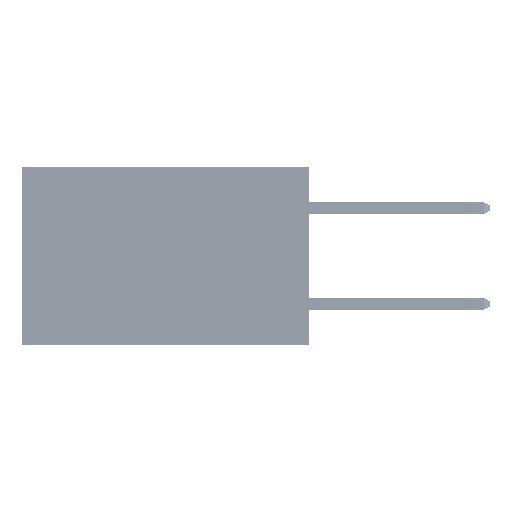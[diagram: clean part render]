
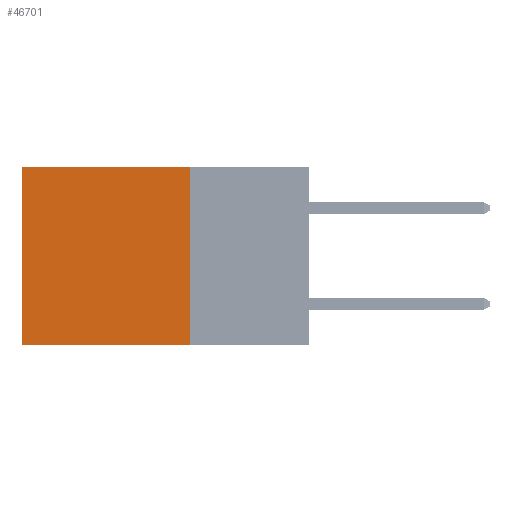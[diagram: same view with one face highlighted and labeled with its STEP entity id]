
A CAD part, left-side view. The second image highlights one B-rep face of the part: STEP entity #46701.
In plain terms, the highlighted planar face has unit normal (-1, 0, 0).
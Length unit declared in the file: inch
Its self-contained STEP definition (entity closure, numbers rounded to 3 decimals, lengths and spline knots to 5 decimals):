
#2729 = DIRECTION ( 'NONE',  ( 0., 0., -1. ) ) ;
#2833 = LINE ( 'NONE', #48284, #40767 ) ;
#3765 = EDGE_CURVE ( 'NONE', #38031, #37282, #28941, .T. ) ;
#4045 = LINE ( 'NONE', #22220, #17287 ) ;
#6251 = DIRECTION ( 'NONE',  ( 0., 0., -1. ) ) ;
#7330 = VERTEX_POINT ( 'NONE', #32236 ) ;
#7373 = VECTOR ( 'NONE', #11178, 39.37008 ) ;
#11178 = DIRECTION ( 'NONE',  ( 0., 1., 0. ) ) ;
#13029 = AXIS2_PLACEMENT_3D ( 'NONE', #47253, #47424, #39059 ) ;
#14104 = EDGE_CURVE ( 'NONE', #38031, #20908, #42827, .T. ) ;
#14466 = ORIENTED_EDGE ( 'NONE', *, *, #3765, .F. ) ;
#15093 = ORIENTED_EDGE ( 'NONE', *, *, #33403, .F. ) ;
#17287 = VECTOR ( 'NONE', #18830, 39.37008 ) ;
#17337 = ORIENTED_EDGE ( 'NONE', *, *, #37130, .T. ) ;
#18830 = DIRECTION ( 'NONE',  ( 0., 1., 0. ) ) ;
#18999 = FACE_OUTER_BOUND ( 'NONE', #23245, .T. ) ;
#19179 = ORIENTED_EDGE ( 'NONE', *, *, #14104, .T. ) ;
#19265 = CARTESIAN_POINT ( 'NONE',  ( 0.2875, 0.6, 0. ) ) ;
#20532 = PLANE ( 'NONE',  #13029 ) ;
#20908 = VERTEX_POINT ( 'NONE', #19265 ) ;
#22220 = CARTESIAN_POINT ( 'NONE',  ( 0.2875, 0.25, -0.37 ) ) ;
#23245 = EDGE_LOOP ( 'NONE', ( #17337, #15093, #14466, #19179 ) ) ;
#25810 = CARTESIAN_POINT ( 'NONE',  ( 0.2875, 0.25, 0. ) ) ;
#28941 = LINE ( 'NONE', #25810, #32562 ) ;
#32236 = CARTESIAN_POINT ( 'NONE',  ( 0.2875, 0.6, -0.37 ) ) ;
#32562 = VECTOR ( 'NONE', #2729, 39.37008 ) ;
#33403 = EDGE_CURVE ( 'NONE', #37282, #7330, #4045, .T. ) ;
#34207 = CARTESIAN_POINT ( 'NONE',  ( 0.2875, 0.25, 0. ) ) ;
#37130 = EDGE_CURVE ( 'NONE', #20908, #7330, #2833, .T. ) ;
#37282 = VERTEX_POINT ( 'NONE', #37897 ) ;
#37897 = CARTESIAN_POINT ( 'NONE',  ( 0.2875, 0.25, -0.37 ) ) ;
#38031 = VERTEX_POINT ( 'NONE', #38105 ) ;
#38105 = CARTESIAN_POINT ( 'NONE',  ( 0.2875, 0.25, 0. ) ) ;
#39059 = DIRECTION ( 'NONE',  ( 0., 0., -1. ) ) ;
#40767 = VECTOR ( 'NONE', #6251, 39.37008 ) ;
#42827 = LINE ( 'NONE', #34207, #7373 ) ;
#46701 = ADVANCED_FACE ( 'NONE', ( #18999 ), #20532, .F. ) ;
#47253 = CARTESIAN_POINT ( 'NONE',  ( 0.2875, 0.25, 0. ) ) ;
#47424 = DIRECTION ( 'NONE',  ( 1., 0., 0. ) ) ;
#48284 = CARTESIAN_POINT ( 'NONE',  ( 0.2875, 0.6, 0. ) ) ;
